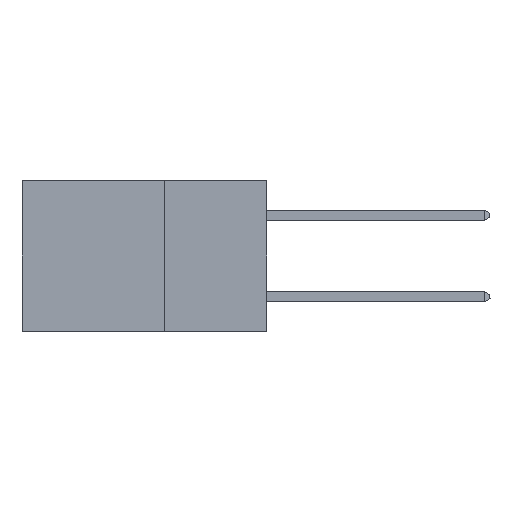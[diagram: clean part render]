
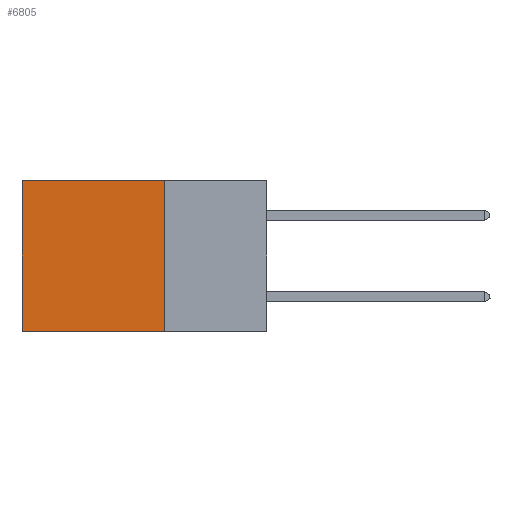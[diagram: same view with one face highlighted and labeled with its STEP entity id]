
A CAD part, left-side view. The second image highlights one B-rep face of the part: STEP entity #6805.
In plain terms, the highlighted planar face has unit normal (-1, 0, 0).
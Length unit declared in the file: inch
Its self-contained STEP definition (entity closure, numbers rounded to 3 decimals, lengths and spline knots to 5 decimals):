
#534 = ORIENTED_EDGE ( 'NONE', *, *, #8052, .T. ) ;
#544 = ORIENTED_EDGE ( 'NONE', *, *, #10477, .T. ) ;
#1055 = PLANE ( 'NONE',  #12693 ) ;
#1302 = LINE ( 'NONE', #13169, #15562 ) ;
#1329 = DIRECTION ( 'NONE',  ( 0., 0., -1. ) ) ;
#2521 = CARTESIAN_POINT ( 'NONE',  ( 0.2875, 0.6, 0. ) ) ;
#2605 = CARTESIAN_POINT ( 'NONE',  ( 0.2875, 0.6, 0. ) ) ;
#3740 = FACE_OUTER_BOUND ( 'NONE', #10636, .T. ) ;
#3743 = CARTESIAN_POINT ( 'NONE',  ( 0.2875, 0.25, 0. ) ) ;
#6633 = VERTEX_POINT ( 'NONE', #10848 ) ;
#6645 = CARTESIAN_POINT ( 'NONE',  ( 0.2875, 0.6, -0.37 ) ) ;
#6805 = ADVANCED_FACE ( 'NONE', ( #3740 ), #1055, .F. ) ;
#6845 = ORIENTED_EDGE ( 'NONE', *, *, #9732, .F. ) ;
#7642 = CARTESIAN_POINT ( 'NONE',  ( 0.2875, 0.25, 0. ) ) ;
#7686 = LINE ( 'NONE', #2521, #14989 ) ;
#8052 = EDGE_CURVE ( 'NONE', #16202, #11925, #10255, .T. ) ;
#8215 = VERTEX_POINT ( 'NONE', #6645 ) ;
#8420 = CARTESIAN_POINT ( 'NONE',  ( 0.2875, 0.25, 0. ) ) ;
#8806 = DIRECTION ( 'NONE',  ( 1., 0., 0. ) ) ;
#8894 = DIRECTION ( 'NONE',  ( 0., 1., 0. ) ) ;
#8898 = ORIENTED_EDGE ( 'NONE', *, *, #12307, .F. ) ;
#9091 = VECTOR ( 'NONE', #1329, 39.37008 ) ;
#9732 = EDGE_CURVE ( 'NONE', #6633, #8215, #1302, .T. ) ;
#10197 = LINE ( 'NONE', #15453, #9091 ) ;
#10255 = LINE ( 'NONE', #3743, #14750 ) ;
#10477 = EDGE_CURVE ( 'NONE', #11925, #8215, #7686, .T. ) ;
#10500 = DIRECTION ( 'NONE',  ( 0., 1., 0. ) ) ;
#10636 = EDGE_LOOP ( 'NONE', ( #544, #6845, #8898, #534 ) ) ;
#10848 = CARTESIAN_POINT ( 'NONE',  ( 0.2875, 0.25, -0.37 ) ) ;
#11454 = DIRECTION ( 'NONE',  ( 0., 0., -1. ) ) ;
#11925 = VERTEX_POINT ( 'NONE', #2605 ) ;
#12307 = EDGE_CURVE ( 'NONE', #16202, #6633, #10197, .T. ) ;
#12693 = AXIS2_PLACEMENT_3D ( 'NONE', #7642, #8806, #13901 ) ;
#13169 = CARTESIAN_POINT ( 'NONE',  ( 0.2875, 0.25, -0.37 ) ) ;
#13901 = DIRECTION ( 'NONE',  ( 0., 0., -1. ) ) ;
#14750 = VECTOR ( 'NONE', #8894, 39.37008 ) ;
#14989 = VECTOR ( 'NONE', #11454, 39.37008 ) ;
#15453 = CARTESIAN_POINT ( 'NONE',  ( 0.2875, 0.25, 0. ) ) ;
#15562 = VECTOR ( 'NONE', #10500, 39.37008 ) ;
#16202 = VERTEX_POINT ( 'NONE', #8420 ) ;
